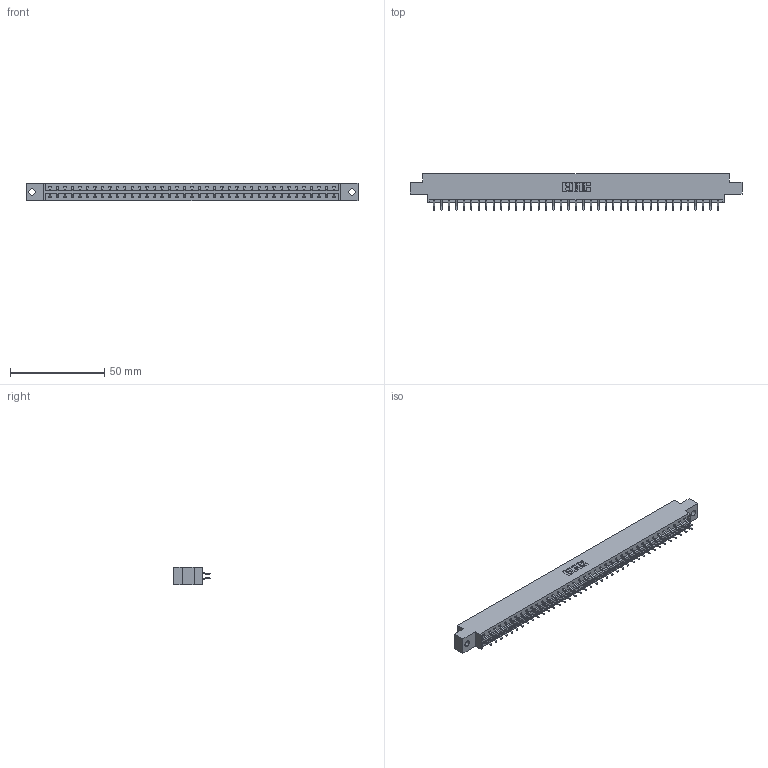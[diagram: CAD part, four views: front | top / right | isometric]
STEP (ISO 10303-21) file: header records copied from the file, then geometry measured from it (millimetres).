
FILE_DESCRIPTION (( 'STEP AP203' ), '1' );
FILE_NAME ('833-078-556-802.STEP', '2020-06-05T20:38:45', ( '' ), ( '' ), 'SwSTEP 2.0', 'SolidWorks 2020', '' );
FILE_SCHEMA (( 'CONFIG_CONTROL_DESIGN' ));
Length unit declared in the file: inch
Products named in the file (3): 345-292-001_556 Tail; 833 Part_Offset - .128 Dia; 833-078-556-802
Assembly tree (79 placements, depth 2):
  833-078-556-802
    833 Part_Offset - .128 Dia
    345-292-001_556 Tail  x78
Bounding box: 176.07 x 19.57 x 9.4 mm (x, y, z)
Volume: 17680.4 mm3; surface area: 20741 mm2
Topology: 79 solids, 79 shells, 4642 faces, 13817 edges, 9106 vertices
Faces by surface type: plane 3194, cylinder 1448
Entity records: 25833 total; most frequent: CARTESIAN_POINT 4302, ORIENTED_EDGE 4226, DIRECTION 3669, EDGE_CURVE 2113, LINE 1977, VECTOR 1977, VERTEX_POINT 1406, AXIS2_PLACEMENT_3D 846
